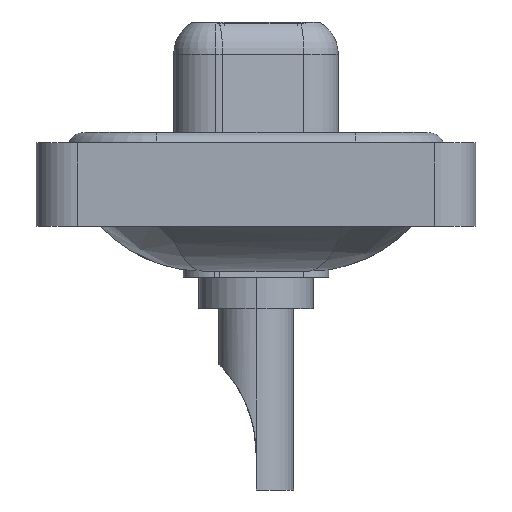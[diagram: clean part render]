
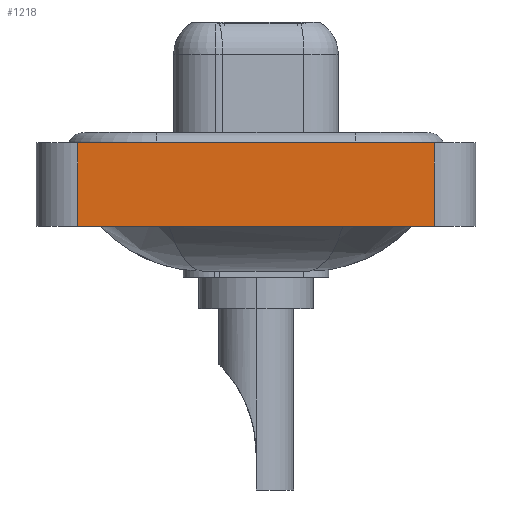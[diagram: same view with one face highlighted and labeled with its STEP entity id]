
A CAD part, left-side view. The second image highlights one B-rep face of the part: STEP entity #1218.
In plain terms, the highlighted planar face has unit normal (-1, 0, 0).
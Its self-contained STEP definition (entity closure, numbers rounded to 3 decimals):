
#725 = VERTEX_POINT ( 'NONE', #10714 ) ;
#1218 = ADVANCED_FACE ( 'NONE', ( #3418 ), #12173, .T. ) ;
#1317 = ORIENTED_EDGE ( 'NONE', *, *, #6621, .F. ) ;
#2066 = ORIENTED_EDGE ( 'NONE', *, *, #12162, .T. ) ;
#2112 = CARTESIAN_POINT ( 'NONE',  ( -7.25, -8.55, -3.6 ) ) ;
#2121 = CARTESIAN_POINT ( 'NONE',  ( -7.25, -8.55, -3.6 ) ) ;
#2243 = LINE ( 'NONE', #16125, #9550 ) ;
#2321 = DIRECTION ( 'NONE',  ( 0., -1., 0. ) ) ;
#3029 = CARTESIAN_POINT ( 'NONE',  ( -7.25, -8.55, 0.4 ) ) ;
#3418 = FACE_OUTER_BOUND ( 'NONE', #3702, .T. ) ;
#3702 = EDGE_LOOP ( 'NONE', ( #2066, #11112, #1317, #11198 ) ) ;
#4212 = LINE ( 'NONE', #7582, #9702 ) ;
#5371 = CARTESIAN_POINT ( 'NONE',  ( -7.25, -8.55, -3.6 ) ) ;
#6621 = EDGE_CURVE ( 'NONE', #10419, #14081, #4212, .T. ) ;
#7582 = CARTESIAN_POINT ( 'NONE',  ( -7.25, 8.55, -3.6 ) ) ;
#8112 = LINE ( 'NONE', #3029, #13913 ) ;
#8183 = DIRECTION ( 'NONE',  ( -1., 0., 0. ) ) ;
#8274 = EDGE_CURVE ( 'NONE', #10419, #9172, #2243, .T. ) ;
#9172 = VERTEX_POINT ( 'NONE', #2112 ) ;
#9550 = VECTOR ( 'NONE', #2321, 1000. ) ;
#9702 = VECTOR ( 'NONE', #12551, 1000. ) ;
#10062 = EDGE_CURVE ( 'NONE', #14081, #725, #8112, .T. ) ;
#10211 = CARTESIAN_POINT ( 'NONE',  ( -7.25, 8.55, 0.4 ) ) ;
#10419 = VERTEX_POINT ( 'NONE', #13232 ) ;
#10706 = DIRECTION ( 'NONE',  ( 0., -1., 0. ) ) ;
#10714 = CARTESIAN_POINT ( 'NONE',  ( -7.25, -8.55, 0.4 ) ) ;
#11112 = ORIENTED_EDGE ( 'NONE', *, *, #10062, .F. ) ;
#11198 = ORIENTED_EDGE ( 'NONE', *, *, #8274, .T. ) ;
#11903 = DIRECTION ( 'NONE',  ( 0., 0., 1. ) ) ;
#11982 = LINE ( 'NONE', #5371, #15522 ) ;
#12162 = EDGE_CURVE ( 'NONE', #9172, #725, #11982, .T. ) ;
#12173 = PLANE ( 'NONE',  #15723 ) ;
#12551 = DIRECTION ( 'NONE',  ( 0., 0., 1. ) ) ;
#13159 = DIRECTION ( 'NONE',  ( 0., 0., 1. ) ) ;
#13232 = CARTESIAN_POINT ( 'NONE',  ( -7.25, 8.55, -3.6 ) ) ;
#13913 = VECTOR ( 'NONE', #10706, 1000. ) ;
#14081 = VERTEX_POINT ( 'NONE', #10211 ) ;
#15522 = VECTOR ( 'NONE', #11903, 1000. ) ;
#15723 = AXIS2_PLACEMENT_3D ( 'NONE', #2121, #8183, #13159 ) ;
#16125 = CARTESIAN_POINT ( 'NONE',  ( -7.25, -8.55, -3.6 ) ) ;
